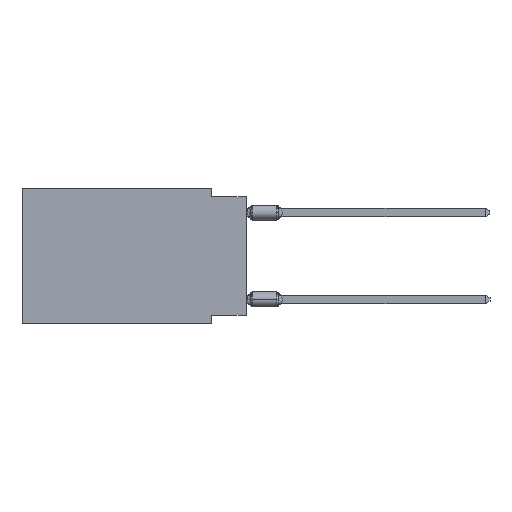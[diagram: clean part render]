
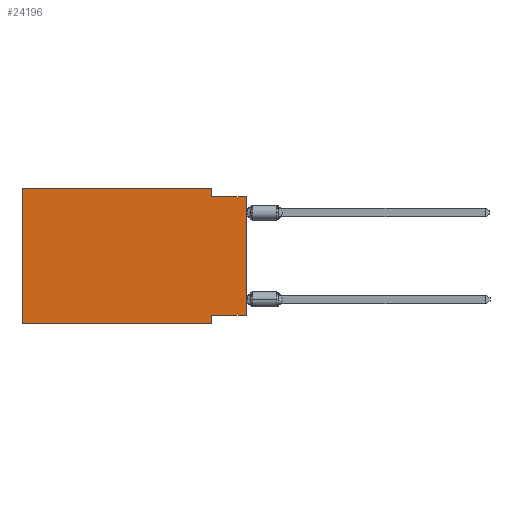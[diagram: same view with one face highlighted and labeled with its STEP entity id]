
A CAD part, left-side view. The second image highlights one B-rep face of the part: STEP entity #24196.
In plain terms, the highlighted planar face has unit normal (-1, 0, 0).
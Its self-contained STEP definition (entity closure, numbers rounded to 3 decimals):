
#542 = LINE ( 'NONE', #16793, #9955 ) ;
#2225 = EDGE_CURVE ( 'NONE', #9902, #11012, #6516, .T. ) ;
#2441 = EDGE_CURVE ( 'NONE', #7576, #26464, #7104, .T. ) ;
#3364 = EDGE_CURVE ( 'NONE', #18933, #18533, #23783, .T. ) ;
#3388 = CARTESIAN_POINT ( 'NONE',  ( 0., 16.383, 0. ) ) ;
#3675 = LINE ( 'NONE', #3388, #12142 ) ;
#4320 = CARTESIAN_POINT ( 'NONE',  ( 0., 16.383, 0. ) ) ;
#4896 = DIRECTION ( 'NONE',  ( 0., 0., -1. ) ) ;
#5424 = LINE ( 'NONE', #21870, #20319 ) ;
#5484 = DIRECTION ( 'NONE',  ( 0., 0., 1. ) ) ;
#5816 = EDGE_CURVE ( 'NONE', #18933, #26464, #18034, .T. ) ;
#6516 = LINE ( 'NONE', #19804, #13131 ) ;
#6993 = DIRECTION ( 'NONE',  ( 0., 0., -1. ) ) ;
#7104 = LINE ( 'NONE', #8897, #10228 ) ;
#7320 = ORIENTED_EDGE ( 'NONE', *, *, #29474, .F. ) ;
#7351 = ORIENTED_EDGE ( 'NONE', *, *, #2225, .T. ) ;
#7576 = VERTEX_POINT ( 'NONE', #8277 ) ;
#7595 = DIRECTION ( 'NONE',  ( 0., -1., 0. ) ) ;
#8277 = CARTESIAN_POINT ( 'NONE',  ( 0., 2.54, -0.635 ) ) ;
#8897 = CARTESIAN_POINT ( 'NONE',  ( 0., 0., -0.635 ) ) ;
#8951 = PLANE ( 'NONE',  #19123 ) ;
#9090 = EDGE_CURVE ( 'NONE', #27816, #26141, #12243, .T. ) ;
#9267 = EDGE_CURVE ( 'NONE', #9902, #27816, #3675, .T. ) ;
#9902 = VERTEX_POINT ( 'NONE', #27893 ) ;
#9955 = VECTOR ( 'NONE', #6993, 1000. ) ;
#10228 = VECTOR ( 'NONE', #20539, 1000. ) ;
#11012 = VERTEX_POINT ( 'NONE', #23863 ) ;
#11231 = VECTOR ( 'NONE', #23636, 1000. ) ;
#11367 = ORIENTED_EDGE ( 'NONE', *, *, #3364, .F. ) ;
#11765 = VECTOR ( 'NONE', #25116, 1000. ) ;
#12142 = VECTOR ( 'NONE', #5484, 1000. ) ;
#12243 = LINE ( 'NONE', #27963, #20343 ) ;
#13131 = VECTOR ( 'NONE', #22515, 1000. ) ;
#14612 = DIRECTION ( 'NONE',  ( 0., 0., -1. ) ) ;
#15104 = CARTESIAN_POINT ( 'NONE',  ( 0., 0., -9.271 ) ) ;
#15305 = CARTESIAN_POINT ( 'NONE',  ( 0., 0., 0. ) ) ;
#15345 = ORIENTED_EDGE ( 'NONE', *, *, #9090, .F. ) ;
#16793 = CARTESIAN_POINT ( 'NONE',  ( 0., 2.54, 0. ) ) ;
#16913 = EDGE_CURVE ( 'NONE', #18533, #11012, #5424, .T. ) ;
#18034 = LINE ( 'NONE', #15305, #11765 ) ;
#18533 = VERTEX_POINT ( 'NONE', #21846 ) ;
#18638 = CARTESIAN_POINT ( 'NONE',  ( 0., 16.383, 0. ) ) ;
#18933 = VERTEX_POINT ( 'NONE', #15104 ) ;
#19123 = AXIS2_PLACEMENT_3D ( 'NONE', #18638, #25569, #4896 ) ;
#19612 = CARTESIAN_POINT ( 'NONE',  ( 0., 0., -0.635 ) ) ;
#19804 = CARTESIAN_POINT ( 'NONE',  ( 0., 16.383, -9.906 ) ) ;
#20319 = VECTOR ( 'NONE', #14612, 1000. ) ;
#20343 = VECTOR ( 'NONE', #7595, 1000. ) ;
#20539 = DIRECTION ( 'NONE',  ( 0., -1., 0. ) ) ;
#21077 = CARTESIAN_POINT ( 'NONE',  ( 0., 0., -9.271 ) ) ;
#21283 = ORIENTED_EDGE ( 'NONE', *, *, #9267, .F. ) ;
#21846 = CARTESIAN_POINT ( 'NONE',  ( 0., 2.54, -9.271 ) ) ;
#21870 = CARTESIAN_POINT ( 'NONE',  ( 0., 2.54, -9.906 ) ) ;
#21880 = ORIENTED_EDGE ( 'NONE', *, *, #2441, .F. ) ;
#22515 = DIRECTION ( 'NONE',  ( 0., -1., 0. ) ) ;
#23153 = FACE_OUTER_BOUND ( 'NONE', #26427, .T. ) ;
#23636 = DIRECTION ( 'NONE',  ( 0., 1., 0. ) ) ;
#23783 = LINE ( 'NONE', #21077, #11231 ) ;
#23863 = CARTESIAN_POINT ( 'NONE',  ( 0., 2.54, -9.906 ) ) ;
#24025 = CARTESIAN_POINT ( 'NONE',  ( 0., 2.54, 0. ) ) ;
#24196 = ADVANCED_FACE ( 'NONE', ( #23153 ), #8951, .F. ) ;
#25116 = DIRECTION ( 'NONE',  ( 0., 0., 1. ) ) ;
#25569 = DIRECTION ( 'NONE',  ( 1., 0., 0. ) ) ;
#26141 = VERTEX_POINT ( 'NONE', #24025 ) ;
#26188 = ORIENTED_EDGE ( 'NONE', *, *, #16913, .F. ) ;
#26427 = EDGE_LOOP ( 'NONE', ( #28661, #21880, #7320, #15345, #21283, #7351, #26188, #11367 ) ) ;
#26464 = VERTEX_POINT ( 'NONE', #19612 ) ;
#27816 = VERTEX_POINT ( 'NONE', #4320 ) ;
#27893 = CARTESIAN_POINT ( 'NONE',  ( 0., 16.383, -9.906 ) ) ;
#27963 = CARTESIAN_POINT ( 'NONE',  ( 0., 16.383, 0. ) ) ;
#28661 = ORIENTED_EDGE ( 'NONE', *, *, #5816, .T. ) ;
#29474 = EDGE_CURVE ( 'NONE', #26141, #7576, #542, .T. ) ;
